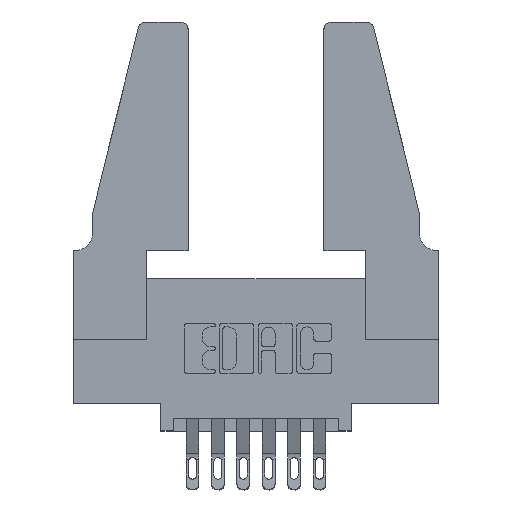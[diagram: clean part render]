
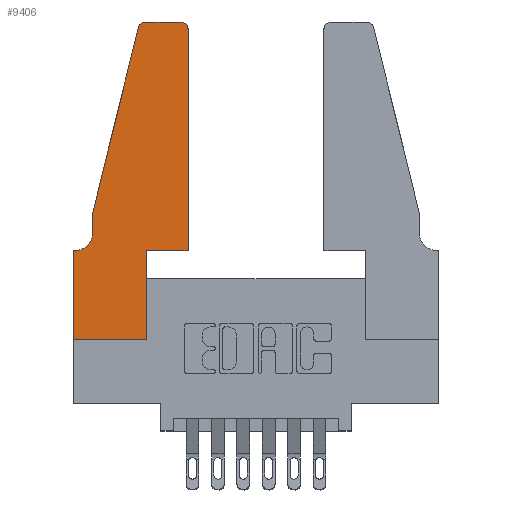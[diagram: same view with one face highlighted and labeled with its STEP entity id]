
A CAD part, top view. The second image highlights one B-rep face of the part: STEP entity #9406.
In plain terms, the highlighted planar face has unit normal (0, 0, 1).
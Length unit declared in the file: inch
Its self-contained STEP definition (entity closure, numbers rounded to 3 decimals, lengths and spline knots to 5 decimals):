
#38 = VECTOR ( 'NONE', #9215, 39.37008 ) ;
#104 = VERTEX_POINT ( 'NONE', #11973 ) ;
#467 = VECTOR ( 'NONE', #2092, 39.37008 ) ;
#728 = LINE ( 'NONE', #11738, #10421 ) ;
#1163 = CARTESIAN_POINT ( 'NONE',  ( 0.4205, 1.25, 0.37 ) ) ;
#1184 = EDGE_CURVE ( 'NONE', #8053, #11983, #12038, .T. ) ;
#1619 = DIRECTION ( 'NONE',  ( -1., 0., 0. ) ) ;
#1738 = CARTESIAN_POINT ( 'NONE',  ( 0.2865, 0., 0.37 ) ) ;
#1756 = CARTESIAN_POINT ( 'NONE',  ( 0.0055, 0.42, 0.37 ) ) ;
#1962 = CIRCLE ( 'NONE', #6904, 0.03 ) ;
#1982 = VERTEX_POINT ( 'NONE', #11534 ) ;
#2092 = DIRECTION ( 'NONE',  ( -0.239, -0.971, 0. ) ) ;
#2299 = EDGE_CURVE ( 'NONE', #11983, #1982, #4149, .T. ) ;
#2664 = VECTOR ( 'NONE', #1619, 39.37008 ) ;
#2763 = DIRECTION ( 'NONE',  ( -1., 0., 0. ) ) ;
#2807 = LINE ( 'NONE', #3693, #38 ) ;
#2912 = EDGE_CURVE ( 'NONE', #9526, #8689, #12126, .T. ) ;
#3145 = VERTEX_POINT ( 'NONE', #8227 ) ;
#3544 = DIRECTION ( 'NONE',  ( 0., 1., 0. ) ) ;
#3588 = CARTESIAN_POINT ( 'NONE',  ( 0.284, 1.22, 0.37 ) ) ;
#3693 = CARTESIAN_POINT ( 'NONE',  ( 0.0755, 0.5, 0.37 ) ) ;
#3769 = EDGE_CURVE ( 'NONE', #8689, #3145, #10707, .T. ) ;
#3876 = VERTEX_POINT ( 'NONE', #7466 ) ;
#3893 = CARTESIAN_POINT ( 'NONE',  ( 0., 0.35, 0.37 ) ) ;
#3927 = EDGE_CURVE ( 'NONE', #3876, #8053, #8988, .T. ) ;
#3947 = CARTESIAN_POINT ( 'NONE',  ( 0., 0., 0.37 ) ) ;
#4125 = VECTOR ( 'NONE', #11154, 39.37008 ) ;
#4149 = LINE ( 'NONE', #8024, #6309 ) ;
#4320 = EDGE_CURVE ( 'NONE', #4745, #104, #2807, .T. ) ;
#4524 = DIRECTION ( 'NONE',  ( 1., 0., 0. ) ) ;
#4700 = CARTESIAN_POINT ( 'NONE',  ( 0.4205, 1.22, 0.37 ) ) ;
#4745 = VERTEX_POINT ( 'NONE', #7032 ) ;
#4770 = VECTOR ( 'NONE', #10386, 39.37008 ) ;
#4809 = CARTESIAN_POINT ( 'NONE',  ( 0., 0., 0.37 ) ) ;
#4836 = DIRECTION ( 'NONE',  ( 0., 0., 1. ) ) ;
#4937 = CARTESIAN_POINT ( 'NONE',  ( 0.0755, 0.5, 0.37 ) ) ;
#5380 = DIRECTION ( 'NONE',  ( -1., 0., 0. ) ) ;
#5607 = DIRECTION ( 'NONE',  ( 1., 0., 0. ) ) ;
#5615 = EDGE_CURVE ( 'NONE', #104, #10705, #7986, .T. ) ;
#5711 = CARTESIAN_POINT ( 'NONE',  ( 0., 0.35, 0.37 ) ) ;
#5729 = CARTESIAN_POINT ( 'NONE',  ( 0.2865, 0.35, 0.37 ) ) ;
#5761 = VERTEX_POINT ( 'NONE', #5711 ) ;
#5803 = EDGE_CURVE ( 'NONE', #5761, #3876, #10806, .T. ) ;
#6221 = DIRECTION ( 'NONE',  ( 1., 0., 0. ) ) ;
#6309 = VECTOR ( 'NONE', #6221, 39.37008 ) ;
#6339 = AXIS2_PLACEMENT_3D ( 'NONE', #3588, #9986, #4524 ) ;
#6852 = EDGE_CURVE ( 'NONE', #11804, #9526, #1962, .T. ) ;
#6904 = AXIS2_PLACEMENT_3D ( 'NONE', #4700, #11083, #5607 ) ;
#7032 = CARTESIAN_POINT ( 'NONE',  ( 0.0755, 0.5, 0.37 ) ) ;
#7223 = LINE ( 'NONE', #11752, #9614 ) ;
#7297 = EDGE_CURVE ( 'NONE', #1982, #11804, #728, .T. ) ;
#7408 = CARTESIAN_POINT ( 'NONE',  ( 0.4505, 1.22, 0.37 ) ) ;
#7466 = CARTESIAN_POINT ( 'NONE',  ( 0., 0., 0.37 ) ) ;
#7986 = CIRCLE ( 'NONE', #9246, 0.07 ) ;
#8024 = CARTESIAN_POINT ( 'NONE',  ( 0.4505, 0.35, 0.37 ) ) ;
#8053 = VERTEX_POINT ( 'NONE', #1738 ) ;
#8227 = CARTESIAN_POINT ( 'NONE',  ( 0.25487, 1.22718, 0.37 ) ) ;
#8232 = ORIENTED_EDGE ( 'NONE', *, *, #2912, .T. ) ;
#8265 = ORIENTED_EDGE ( 'NONE', *, *, #3769, .T. ) ;
#8292 = DIRECTION ( 'NONE',  ( 0., 0., -1. ) ) ;
#8301 = ORIENTED_EDGE ( 'NONE', *, *, #10117, .T. ) ;
#8403 = VECTOR ( 'NONE', #9472, 39.37008 ) ;
#8689 = VERTEX_POINT ( 'NONE', #11085 ) ;
#8912 = AXIS2_PLACEMENT_3D ( 'NONE', #3893, #4836, #11232 ) ;
#8988 = LINE ( 'NONE', #4809, #4125 ) ;
#9034 = ORIENTED_EDGE ( 'NONE', *, *, #4320, .T. ) ;
#9094 = FACE_OUTER_BOUND ( 'NONE', #10067, .T. ) ;
#9215 = DIRECTION ( 'NONE',  ( 0., -1., 0. ) ) ;
#9246 = AXIS2_PLACEMENT_3D ( 'NONE', #1756, #8292, #2763 ) ;
#9256 = ORIENTED_EDGE ( 'NONE', *, *, #5615, .T. ) ;
#9371 = ORIENTED_EDGE ( 'NONE', *, *, #11546, .T. ) ;
#9406 = ADVANCED_FACE ( 'NONE', ( #9094 ), #10281, .T. ) ;
#9433 = ORIENTED_EDGE ( 'NONE', *, *, #5803, .T. ) ;
#9443 = ORIENTED_EDGE ( 'NONE', *, *, #3927, .T. ) ;
#9472 = DIRECTION ( 'NONE',  ( 0., -1., 0. ) ) ;
#9500 = ORIENTED_EDGE ( 'NONE', *, *, #1184, .T. ) ;
#9526 = VERTEX_POINT ( 'NONE', #1163 ) ;
#9614 = VECTOR ( 'NONE', #5380, 39.37008 ) ;
#9620 = ORIENTED_EDGE ( 'NONE', *, *, #2299, .T. ) ;
#9670 = ORIENTED_EDGE ( 'NONE', *, *, #7297, .T. ) ;
#9694 = ORIENTED_EDGE ( 'NONE', *, *, #6852, .T. ) ;
#9986 = DIRECTION ( 'NONE',  ( 0., 0., 1. ) ) ;
#10067 = EDGE_LOOP ( 'NONE', ( #8232, #8265, #8301, #9034, #9256, #9371, #9433, #9443, #9500, #9620, #9670, #9694 ) ) ;
#10117 = EDGE_CURVE ( 'NONE', #3145, #4745, #10490, .T. ) ;
#10281 = PLANE ( 'NONE',  #8912 ) ;
#10331 = CARTESIAN_POINT ( 'NONE',  ( 0.0055, 0.35, 0.37 ) ) ;
#10386 = DIRECTION ( 'NONE',  ( 0., 1., 0. ) ) ;
#10421 = VECTOR ( 'NONE', #3544, 39.37008 ) ;
#10490 = LINE ( 'NONE', #4937, #467 ) ;
#10705 = VERTEX_POINT ( 'NONE', #10331 ) ;
#10707 = CIRCLE ( 'NONE', #6339, 0.03 ) ;
#10806 = LINE ( 'NONE', #3947, #8403 ) ;
#11083 = DIRECTION ( 'NONE',  ( 0., 0., 1. ) ) ;
#11085 = CARTESIAN_POINT ( 'NONE',  ( 0.284, 1.25, 0.37 ) ) ;
#11154 = DIRECTION ( 'NONE',  ( 1., 0., 0. ) ) ;
#11232 = DIRECTION ( 'NONE',  ( 1., 0., 0. ) ) ;
#11306 = CARTESIAN_POINT ( 'NONE',  ( 0.2865, 0.35, 0.37 ) ) ;
#11534 = CARTESIAN_POINT ( 'NONE',  ( 0.4505, 0.35, 0.37 ) ) ;
#11546 = EDGE_CURVE ( 'NONE', #10705, #5761, #7223, .T. ) ;
#11738 = CARTESIAN_POINT ( 'NONE',  ( 0.4505, 0.35, 0.37 ) ) ;
#11752 = CARTESIAN_POINT ( 'NONE',  ( 0.0755, 0.35, 0.37 ) ) ;
#11804 = VERTEX_POINT ( 'NONE', #7408 ) ;
#11865 = CARTESIAN_POINT ( 'NONE',  ( 0.2605, 1.25, 0.37 ) ) ;
#11973 = CARTESIAN_POINT ( 'NONE',  ( 0.0755, 0.42, 0.37 ) ) ;
#11983 = VERTEX_POINT ( 'NONE', #11306 ) ;
#12038 = LINE ( 'NONE', #5729, #4770 ) ;
#12126 = LINE ( 'NONE', #11865, #2664 ) ;
